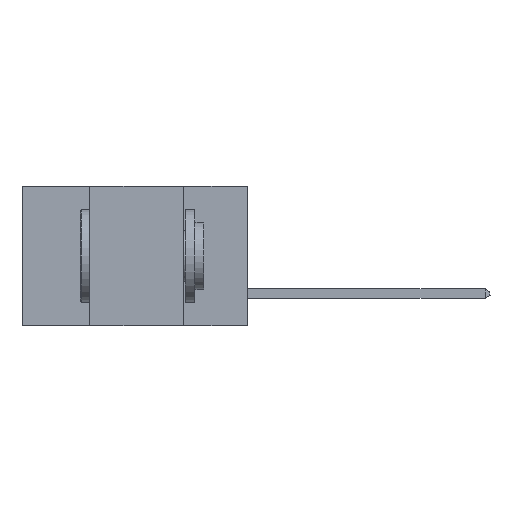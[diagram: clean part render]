
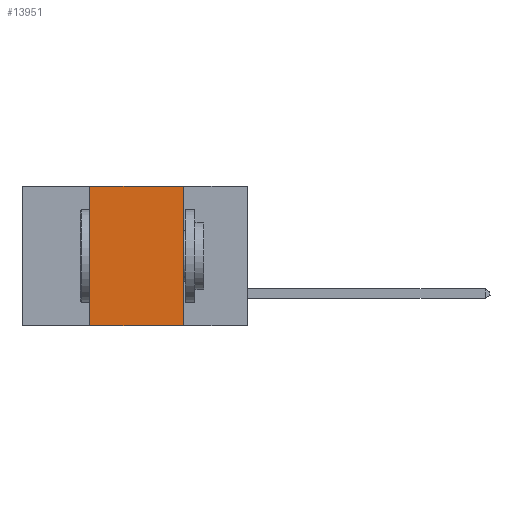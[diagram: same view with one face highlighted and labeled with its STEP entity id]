
A CAD part, left-side view. The second image highlights one B-rep face of the part: STEP entity #13951.
In plain terms, the highlighted planar face has unit normal (-1, 0, 0).
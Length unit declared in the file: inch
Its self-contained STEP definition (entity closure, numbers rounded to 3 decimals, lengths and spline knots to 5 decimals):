
#296 = EDGE_CURVE ( 'NONE', #19791, #13018, #19043, .T. ) ;
#299 = PLANE ( 'NONE',  #18305 ) ;
#534 = EDGE_CURVE ( 'NONE', #2545, #13876, #12914, .T. ) ;
#926 = LINE ( 'NONE', #20144, #13014 ) ;
#2508 = LINE ( 'NONE', #19562, #19732 ) ;
#2545 = VERTEX_POINT ( 'NONE', #16363 ) ;
#2620 = EDGE_CURVE ( 'NONE', #13876, #19791, #2508, .T. ) ;
#2768 = ORIENTED_EDGE ( 'NONE', *, *, #534, .F. ) ;
#4936 = EDGE_CURVE ( 'NONE', #2545, #13018, #926, .T. ) ;
#5261 = DIRECTION ( 'NONE',  ( 1., 0., 0. ) ) ;
#5321 = CARTESIAN_POINT ( 'NONE',  ( 0., 0.17, 0. ) ) ;
#8256 = ORIENTED_EDGE ( 'NONE', *, *, #4936, .T. ) ;
#8372 = CARTESIAN_POINT ( 'NONE',  ( 0., 0.6, 0. ) ) ;
#9736 = EDGE_LOOP ( 'NONE', ( #17285, #17530, #2768, #8256 ) ) ;
#11139 = CARTESIAN_POINT ( 'NONE',  ( 0., 0.42, 0. ) ) ;
#11531 = DIRECTION ( 'NONE',  ( 0., -1., 0. ) ) ;
#12163 = DIRECTION ( 'NONE',  ( 0., -1., 0. ) ) ;
#12914 = LINE ( 'NONE', #19098, #16622 ) ;
#13014 = VECTOR ( 'NONE', #12163, 39.37008 ) ;
#13018 = VERTEX_POINT ( 'NONE', #18054 ) ;
#13876 = VERTEX_POINT ( 'NONE', #11139 ) ;
#13891 = VECTOR ( 'NONE', #16341, 39.37008 ) ;
#13951 = ADVANCED_FACE ( 'NONE', ( #17964 ), #299, .F. ) ;
#16341 = DIRECTION ( 'NONE',  ( 0., 0., -1. ) ) ;
#16363 = CARTESIAN_POINT ( 'NONE',  ( 0., 0.42, -0.37 ) ) ;
#16622 = VECTOR ( 'NONE', #18899, 39.37008 ) ;
#17285 = ORIENTED_EDGE ( 'NONE', *, *, #296, .F. ) ;
#17530 = ORIENTED_EDGE ( 'NONE', *, *, #2620, .F. ) ;
#17764 = DIRECTION ( 'NONE',  ( 0., 0., -1. ) ) ;
#17964 = FACE_OUTER_BOUND ( 'NONE', #9736, .T. ) ;
#18054 = CARTESIAN_POINT ( 'NONE',  ( 0., 0.17, -0.37 ) ) ;
#18305 = AXIS2_PLACEMENT_3D ( 'NONE', #8372, #5261, #17764 ) ;
#18899 = DIRECTION ( 'NONE',  ( 0., 0., 1. ) ) ;
#19043 = LINE ( 'NONE', #5321, #13891 ) ;
#19098 = CARTESIAN_POINT ( 'NONE',  ( 0., 0.42, 0. ) ) ;
#19243 = CARTESIAN_POINT ( 'NONE',  ( 0., 0.17, 0. ) ) ;
#19562 = CARTESIAN_POINT ( 'NONE',  ( 0., 0.6, 0. ) ) ;
#19732 = VECTOR ( 'NONE', #11531, 39.37008 ) ;
#19791 = VERTEX_POINT ( 'NONE', #19243 ) ;
#20144 = CARTESIAN_POINT ( 'NONE',  ( 0., 0.6, -0.37 ) ) ;
